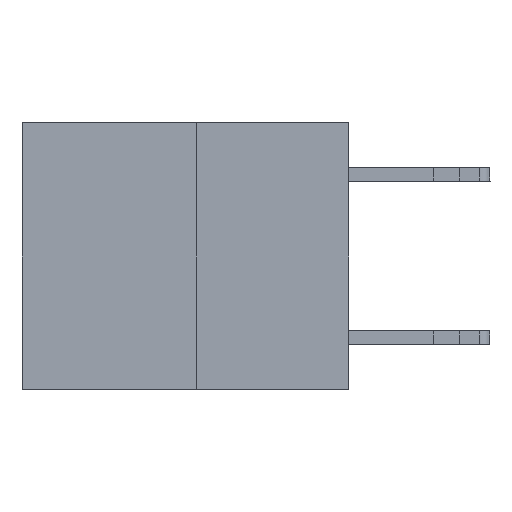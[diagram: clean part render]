
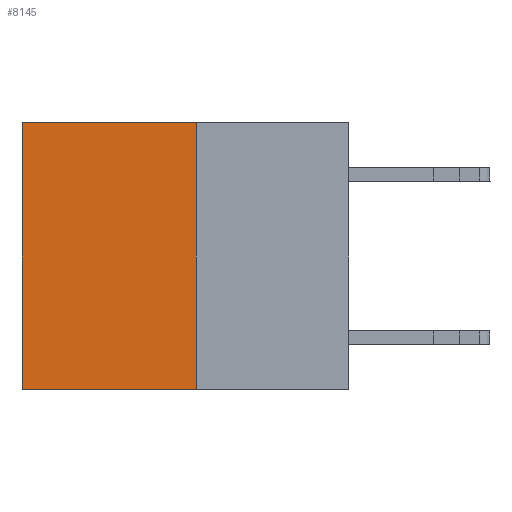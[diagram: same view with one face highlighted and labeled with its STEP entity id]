
A CAD part, left-side view. The second image highlights one B-rep face of the part: STEP entity #8145.
In plain terms, the highlighted planar face has unit normal (-1, 0, 0).
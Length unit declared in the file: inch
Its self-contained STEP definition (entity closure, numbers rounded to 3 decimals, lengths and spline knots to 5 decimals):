
#14 = ORIENTED_EDGE ( 'NONE', *, *, #12374, .F. ) ;
#260 = CARTESIAN_POINT ( 'NONE',  ( 0.3165, 0.6, -0.49 ) ) ;
#779 = FACE_OUTER_BOUND ( 'NONE', #1563, .T. ) ;
#897 = VECTOR ( 'NONE', #23162, 39.37008 ) ;
#1005 = DIRECTION ( 'NONE',  ( 0., 0., -1. ) ) ;
#1283 = VERTEX_POINT ( 'NONE', #21797 ) ;
#1307 = VERTEX_POINT ( 'NONE', #260 ) ;
#1563 = EDGE_LOOP ( 'NONE', ( #19216, #21024, #14, #14957 ) ) ;
#1809 = DIRECTION ( 'NONE',  ( 0., 0., -1. ) ) ;
#2282 = PLANE ( 'NONE',  #16344 ) ;
#2658 = EDGE_CURVE ( 'NONE', #8064, #1307, #3002, .T. ) ;
#3002 = LINE ( 'NONE', #19942, #4412 ) ;
#3740 = LINE ( 'NONE', #16281, #897 ) ;
#4253 = VECTOR ( 'NONE', #1005, 39.37008 ) ;
#4412 = VECTOR ( 'NONE', #12791, 39.37008 ) ;
#5678 = DIRECTION ( 'NONE',  ( 1., 0., 0. ) ) ;
#6800 = VERTEX_POINT ( 'NONE', #23205 ) ;
#7432 = CARTESIAN_POINT ( 'NONE',  ( 0.3165, 0.28, -0.49 ) ) ;
#8064 = VERTEX_POINT ( 'NONE', #9365 ) ;
#8145 = ADVANCED_FACE ( 'NONE', ( #779 ), #2282, .F. ) ;
#9182 = CARTESIAN_POINT ( 'NONE',  ( 0.3165, 0.6, -0.49 ) ) ;
#9365 = CARTESIAN_POINT ( 'NONE',  ( 0.3165, 0.28, -0.49 ) ) ;
#11431 = LINE ( 'NONE', #9182, #20763 ) ;
#12374 = EDGE_CURVE ( 'NONE', #6800, #8064, #14967, .T. ) ;
#12791 = DIRECTION ( 'NONE',  ( 0., 1., 0. ) ) ;
#14957 = ORIENTED_EDGE ( 'NONE', *, *, #15784, .T. ) ;
#14967 = LINE ( 'NONE', #22650, #4253 ) ;
#15784 = EDGE_CURVE ( 'NONE', #6800, #1283, #3740, .T. ) ;
#16281 = CARTESIAN_POINT ( 'NONE',  ( 0.3165, 0.28, 0. ) ) ;
#16344 = AXIS2_PLACEMENT_3D ( 'NONE', #7432, #5678, #18318 ) ;
#18318 = DIRECTION ( 'NONE',  ( 0., 0., -1. ) ) ;
#19216 = ORIENTED_EDGE ( 'NONE', *, *, #22393, .T. ) ;
#19942 = CARTESIAN_POINT ( 'NONE',  ( 0.3165, 0.28, -0.49 ) ) ;
#20763 = VECTOR ( 'NONE', #1809, 39.37008 ) ;
#21024 = ORIENTED_EDGE ( 'NONE', *, *, #2658, .F. ) ;
#21797 = CARTESIAN_POINT ( 'NONE',  ( 0.3165, 0.6, 0. ) ) ;
#22393 = EDGE_CURVE ( 'NONE', #1283, #1307, #11431, .T. ) ;
#22650 = CARTESIAN_POINT ( 'NONE',  ( 0.3165, 0.28, -0.49 ) ) ;
#23162 = DIRECTION ( 'NONE',  ( 0., 1., 0. ) ) ;
#23205 = CARTESIAN_POINT ( 'NONE',  ( 0.3165, 0.28, 0. ) ) ;
